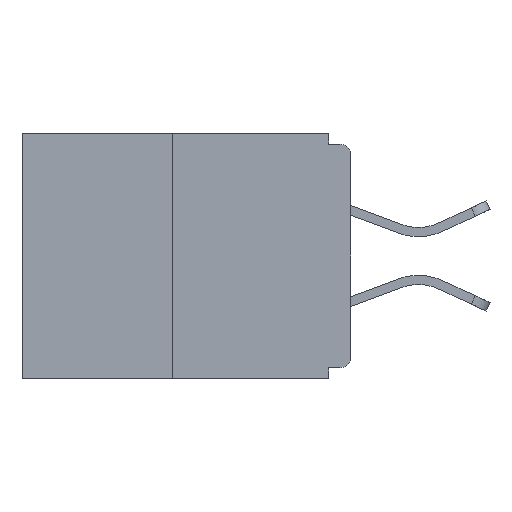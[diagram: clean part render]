
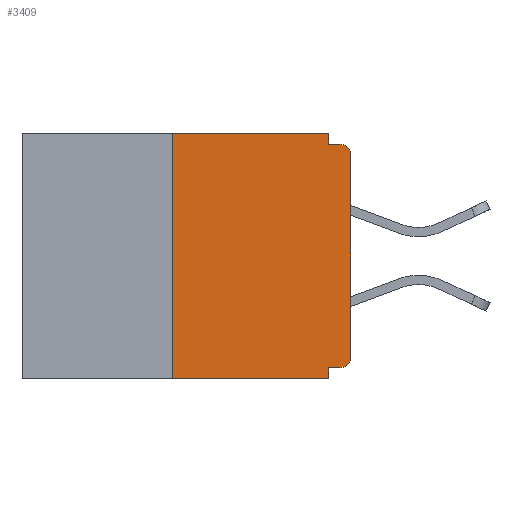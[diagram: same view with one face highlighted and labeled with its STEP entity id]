
A CAD part, left-side view. The second image highlights one B-rep face of the part: STEP entity #3409.
In plain terms, the highlighted planar face has unit normal (-1, 0, 0).
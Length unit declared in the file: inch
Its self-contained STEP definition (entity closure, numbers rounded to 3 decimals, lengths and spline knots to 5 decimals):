
#162 = DIRECTION ( 'NONE',  ( 0., 0., -1. ) ) ;
#229 = CARTESIAN_POINT ( 'NONE',  ( 0., 0., 0. ) ) ;
#293 = EDGE_CURVE ( 'NONE', #10982, #15053, #18428, .T. ) ;
#1102 = EDGE_CURVE ( 'NONE', #19591, #5834, #2275, .T. ) ;
#1295 = CIRCLE ( 'NONE', #11150, 0.015 ) ;
#1418 = VECTOR ( 'NONE', #13807, 39.37008 ) ;
#1994 = ORIENTED_EDGE ( 'NONE', *, *, #4603, .F. ) ;
#2133 = ORIENTED_EDGE ( 'NONE', *, *, #3378, .T. ) ;
#2275 = LINE ( 'NONE', #8891, #1418 ) ;
#2401 = DIRECTION ( 'NONE',  ( 0., -1., 0. ) ) ;
#2494 = CARTESIAN_POINT ( 'NONE',  ( 0., 0., -0.03 ) ) ;
#2951 = ORIENTED_EDGE ( 'NONE', *, *, #10978, .T. ) ;
#3378 = EDGE_CURVE ( 'NONE', #13813, #18559, #5989, .T. ) ;
#3409 = ADVANCED_FACE ( 'NONE', ( #9916 ), #9698, .F. ) ;
#3426 = CARTESIAN_POINT ( 'NONE',  ( 0., 0., -0.313 ) ) ;
#3546 = ORIENTED_EDGE ( 'NONE', *, *, #17896, .F. ) ;
#3858 = CARTESIAN_POINT ( 'NONE',  ( 0., 0.031, -0.343 ) ) ;
#4603 = EDGE_CURVE ( 'NONE', #13813, #10982, #16042, .T. ) ;
#4660 = DIRECTION ( 'NONE',  ( 0., 0., -1. ) ) ;
#4854 = EDGE_CURVE ( 'NONE', #18559, #16224, #13140, .T. ) ;
#4984 = ORIENTED_EDGE ( 'NONE', *, *, #5790, .F. ) ;
#5667 = VECTOR ( 'NONE', #12714, 39.37008 ) ;
#5790 = EDGE_CURVE ( 'NONE', #14706, #18916, #7134, .T. ) ;
#5834 = VERTEX_POINT ( 'NONE', #20751 ) ;
#5989 = CIRCLE ( 'NONE', #9418, 0.015 ) ;
#7134 = LINE ( 'NONE', #13667, #16150 ) ;
#7709 = DIRECTION ( 'NONE',  ( 0., -1., 0. ) ) ;
#8191 = DIRECTION ( 'NONE',  ( 1., 0., 0. ) ) ;
#8339 = EDGE_CURVE ( 'NONE', #5834, #13020, #19260, .T. ) ;
#8891 = CARTESIAN_POINT ( 'NONE',  ( 0., 0.031, 0. ) ) ;
#9250 = VECTOR ( 'NONE', #9827, 39.37008 ) ;
#9418 = AXIS2_PLACEMENT_3D ( 'NONE', #13110, #16329, #4660 ) ;
#9687 = EDGE_CURVE ( 'NONE', #16224, #13020, #1295, .T. ) ;
#9698 = PLANE ( 'NONE',  #17973 ) ;
#9827 = DIRECTION ( 'NONE',  ( 0., 0., 1. ) ) ;
#9916 = FACE_OUTER_BOUND ( 'NONE', #16872, .T. ) ;
#10413 = LINE ( 'NONE', #16742, #11960 ) ;
#10819 = LINE ( 'NONE', #20589, #13268 ) ;
#10978 = EDGE_CURVE ( 'NONE', #14706, #15053, #10819, .T. ) ;
#10982 = VERTEX_POINT ( 'NONE', #20809 ) ;
#10996 = ORIENTED_EDGE ( 'NONE', *, *, #1102, .F. ) ;
#11150 = AXIS2_PLACEMENT_3D ( 'NONE', #18963, #20356, #13811 ) ;
#11182 = CARTESIAN_POINT ( 'NONE',  ( 0., 0.46, 0. ) ) ;
#11664 = VECTOR ( 'NONE', #162, 39.37008 ) ;
#11960 = VECTOR ( 'NONE', #2401, 39.37008 ) ;
#12714 = DIRECTION ( 'NONE',  ( 0., 1., 0. ) ) ;
#12759 = ORIENTED_EDGE ( 'NONE', *, *, #9687, .T. ) ;
#13020 = VERTEX_POINT ( 'NONE', #18201 ) ;
#13110 = CARTESIAN_POINT ( 'NONE',  ( 0., 0.015, -0.313 ) ) ;
#13140 = LINE ( 'NONE', #229, #9250 ) ;
#13268 = VECTOR ( 'NONE', #7709, 39.37008 ) ;
#13666 = CARTESIAN_POINT ( 'NONE',  ( 0., 0.015, -0.328 ) ) ;
#13667 = CARTESIAN_POINT ( 'NONE',  ( 0., 0.25, 0. ) ) ;
#13807 = DIRECTION ( 'NONE',  ( 0., 0., -1. ) ) ;
#13811 = DIRECTION ( 'NONE',  ( 0., 0., -1. ) ) ;
#13813 = VERTEX_POINT ( 'NONE', #13666 ) ;
#13902 = VECTOR ( 'NONE', #15913, 39.37008 ) ;
#14143 = CARTESIAN_POINT ( 'NONE',  ( 0., 0.25, -0.343 ) ) ;
#14706 = VERTEX_POINT ( 'NONE', #14143 ) ;
#14865 = ORIENTED_EDGE ( 'NONE', *, *, #293, .F. ) ;
#15031 = ORIENTED_EDGE ( 'NONE', *, *, #4854, .T. ) ;
#15053 = VERTEX_POINT ( 'NONE', #15465 ) ;
#15465 = CARTESIAN_POINT ( 'NONE',  ( 0., 0.031, -0.343 ) ) ;
#15913 = DIRECTION ( 'NONE',  ( 0., -1., 0. ) ) ;
#16042 = LINE ( 'NONE', #20781, #5667 ) ;
#16150 = VECTOR ( 'NONE', #20220, 39.37008 ) ;
#16224 = VERTEX_POINT ( 'NONE', #2494 ) ;
#16329 = DIRECTION ( 'NONE',  ( -1., 0., 0. ) ) ;
#16441 = DIRECTION ( 'NONE',  ( 0., 0., -1. ) ) ;
#16742 = CARTESIAN_POINT ( 'NONE',  ( 0., 0.46, 0. ) ) ;
#16872 = EDGE_LOOP ( 'NONE', ( #3546, #4984, #2951, #14865, #1994, #2133, #15031, #12759, #19375, #10996 ) ) ;
#17896 = EDGE_CURVE ( 'NONE', #18916, #19591, #10413, .T. ) ;
#17973 = AXIS2_PLACEMENT_3D ( 'NONE', #11182, #8191, #16441 ) ;
#18201 = CARTESIAN_POINT ( 'NONE',  ( 0., 0.015, -0.015 ) ) ;
#18428 = LINE ( 'NONE', #3858, #11664 ) ;
#18559 = VERTEX_POINT ( 'NONE', #3426 ) ;
#18916 = VERTEX_POINT ( 'NONE', #20761 ) ;
#18963 = CARTESIAN_POINT ( 'NONE',  ( 0., 0.015, -0.03 ) ) ;
#19260 = LINE ( 'NONE', #20883, #13902 ) ;
#19375 = ORIENTED_EDGE ( 'NONE', *, *, #8339, .F. ) ;
#19591 = VERTEX_POINT ( 'NONE', #21034 ) ;
#20220 = DIRECTION ( 'NONE',  ( 0., 0., 1. ) ) ;
#20356 = DIRECTION ( 'NONE',  ( -1., 0., 0. ) ) ;
#20589 = CARTESIAN_POINT ( 'NONE',  ( 0., 0.46, -0.343 ) ) ;
#20751 = CARTESIAN_POINT ( 'NONE',  ( 0., 0.031, -0.015 ) ) ;
#20761 = CARTESIAN_POINT ( 'NONE',  ( 0., 0.25, 0. ) ) ;
#20781 = CARTESIAN_POINT ( 'NONE',  ( 0., 0., -0.328 ) ) ;
#20809 = CARTESIAN_POINT ( 'NONE',  ( 0., 0.031, -0.328 ) ) ;
#20883 = CARTESIAN_POINT ( 'NONE',  ( 0., 0., -0.015 ) ) ;
#21034 = CARTESIAN_POINT ( 'NONE',  ( 0., 0.031, 0. ) ) ;
